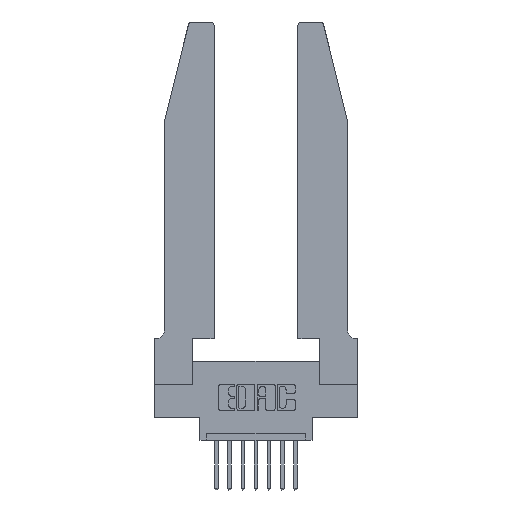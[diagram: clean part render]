
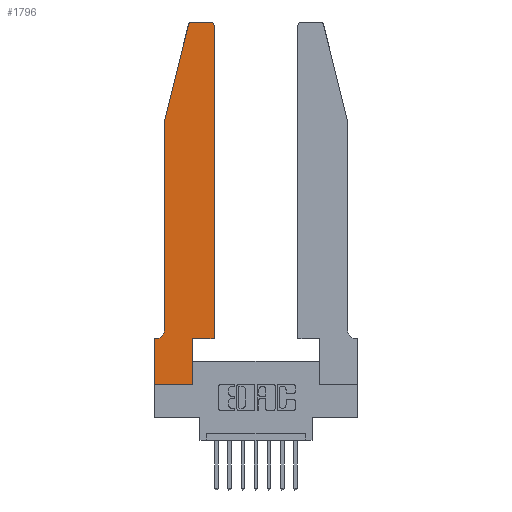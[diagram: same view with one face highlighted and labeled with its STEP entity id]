
A CAD part, top view. The second image highlights one B-rep face of the part: STEP entity #1796.
In plain terms, the highlighted planar face has unit normal (0, 0, 1).
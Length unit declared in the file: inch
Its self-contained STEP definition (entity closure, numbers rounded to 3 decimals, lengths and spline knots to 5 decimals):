
#229 = ORIENTED_EDGE ( 'NONE', *, *, #1550, .T. ) ;
#230 = DIRECTION ( 'NONE',  ( 1., 0., 0. ) ) ;
#375 = EDGE_CURVE ( 'NONE', #14135, #950, #12281, .T. ) ;
#395 = DIRECTION ( 'NONE',  ( 0., 1., 0. ) ) ;
#457 = AXIS2_PLACEMENT_3D ( 'NONE', #3667, #13935, #230 ) ;
#546 = CARTESIAN_POINT ( 'NONE',  ( 0.4505, 0.35, 0.37 ) ) ;
#648 = EDGE_CURVE ( 'NONE', #1232, #12059, #10456, .T. ) ;
#710 = ORIENTED_EDGE ( 'NONE', *, *, #1595, .T. ) ;
#726 = DIRECTION ( 'NONE',  ( 1., 0., 0. ) ) ;
#830 = CARTESIAN_POINT ( 'NONE',  ( 0.4505, 2.72, 0.37 ) ) ;
#925 = DIRECTION ( 'NONE',  ( 0., 0., -1. ) ) ;
#950 = VERTEX_POINT ( 'NONE', #11310 ) ;
#986 = DIRECTION ( 'NONE',  ( 1., 0., 0. ) ) ;
#1047 = DIRECTION ( 'NONE',  ( -1., 0., 0. ) ) ;
#1192 = DIRECTION ( 'NONE',  ( 0., -1., 0. ) ) ;
#1232 = VERTEX_POINT ( 'NONE', #3815 ) ;
#1277 = ORIENTED_EDGE ( 'NONE', *, *, #648, .T. ) ;
#1492 = PLANE ( 'NONE',  #457 ) ;
#1550 = EDGE_CURVE ( 'NONE', #12592, #5306, #10961, .T. ) ;
#1595 = EDGE_CURVE ( 'NONE', #950, #5706, #12934, .T. ) ;
#1796 = ADVANCED_FACE ( 'NONE', ( #2168 ), #1492, .T. ) ;
#1823 = DIRECTION ( 'NONE',  ( -1., 0., 0. ) ) ;
#1862 = EDGE_CURVE ( 'NONE', #3837, #14767, #1971, .T. ) ;
#1971 = CIRCLE ( 'NONE', #5374, 0.03 ) ;
#2168 = FACE_OUTER_BOUND ( 'NONE', #11415, .T. ) ;
#2303 = CARTESIAN_POINT ( 'NONE',  ( 0.284, 2.75, 0.37 ) ) ;
#2706 = DIRECTION ( 'NONE',  ( 0., 0., 1. ) ) ;
#2870 = ORIENTED_EDGE ( 'NONE', *, *, #4803, .T. ) ;
#2921 = LINE ( 'NONE', #11728, #12466 ) ;
#3088 = CIRCLE ( 'NONE', #8132, 0.07 ) ;
#3297 = VECTOR ( 'NONE', #1823, 39.37008 ) ;
#3367 = VECTOR ( 'NONE', #726, 39.37008 ) ;
#3453 = EDGE_CURVE ( 'NONE', #5306, #11946, #10013, .T. ) ;
#3667 = CARTESIAN_POINT ( 'NONE',  ( 0., 0.35, 0.37 ) ) ;
#3739 = DIRECTION ( 'NONE',  ( -0.239, -0.971, 0. ) ) ;
#3809 = VECTOR ( 'NONE', #3739, 39.37008 ) ;
#3815 = CARTESIAN_POINT ( 'NONE',  ( 0.25487, 2.72718, 0.37 ) ) ;
#3837 = VERTEX_POINT ( 'NONE', #830 ) ;
#3891 = ORIENTED_EDGE ( 'NONE', *, *, #8938, .T. ) ;
#4136 = VECTOR ( 'NONE', #8651, 39.37008 ) ;
#4215 = CIRCLE ( 'NONE', #12086, 0.03 ) ;
#4458 = DIRECTION ( 'NONE',  ( 1., 0., 0. ) ) ;
#4609 = ORIENTED_EDGE ( 'NONE', *, *, #3453, .T. ) ;
#4619 = VECTOR ( 'NONE', #395, 39.37008 ) ;
#4803 = EDGE_CURVE ( 'NONE', #11946, #3837, #7689, .T. ) ;
#4971 = LINE ( 'NONE', #10014, #3367 ) ;
#5232 = ORIENTED_EDGE ( 'NONE', *, *, #13812, .T. ) ;
#5306 = VERTEX_POINT ( 'NONE', #6312 ) ;
#5374 = AXIS2_PLACEMENT_3D ( 'NONE', #14140, #2706, #6211 ) ;
#5556 = CARTESIAN_POINT ( 'NONE',  ( 0.4505, 0.35, 0.37 ) ) ;
#5706 = VERTEX_POINT ( 'NONE', #10268 ) ;
#5833 = VERTEX_POINT ( 'NONE', #10664 ) ;
#6033 = CARTESIAN_POINT ( 'NONE',  ( 0.0755, 2., 0.37 ) ) ;
#6211 = DIRECTION ( 'NONE',  ( 1., 0., 0. ) ) ;
#6312 = CARTESIAN_POINT ( 'NONE',  ( 0.2865, 0.35, 0.37 ) ) ;
#6602 = VECTOR ( 'NONE', #986, 39.37008 ) ;
#6753 = VERTEX_POINT ( 'NONE', #2303 ) ;
#6774 = ORIENTED_EDGE ( 'NONE', *, *, #1862, .T. ) ;
#6819 = CARTESIAN_POINT ( 'NONE',  ( 0., 0., 0.37 ) ) ;
#7458 = CARTESIAN_POINT ( 'NONE',  ( 0.2865, 0., 0.37 ) ) ;
#7612 = EDGE_CURVE ( 'NONE', #14767, #6753, #10496, .T. ) ;
#7613 = EDGE_CURVE ( 'NONE', #6753, #1232, #4215, .T. ) ;
#7689 = LINE ( 'NONE', #546, #4619 ) ;
#8132 = AXIS2_PLACEMENT_3D ( 'NONE', #8798, #925, #14589 ) ;
#8651 = DIRECTION ( 'NONE',  ( 0., 1., 0. ) ) ;
#8798 = CARTESIAN_POINT ( 'NONE',  ( 0.0055, 0.42, 0.37 ) ) ;
#8938 = EDGE_CURVE ( 'NONE', #12059, #5833, #2921, .T. ) ;
#9040 = CARTESIAN_POINT ( 'NONE',  ( 0.2605, 2.75, 0.37 ) ) ;
#10013 = LINE ( 'NONE', #5556, #6602 ) ;
#10014 = CARTESIAN_POINT ( 'NONE',  ( 0., 0., 0.37 ) ) ;
#10268 = CARTESIAN_POINT ( 'NONE',  ( 0., 0., 0.37 ) ) ;
#10456 = LINE ( 'NONE', #10603, #3809 ) ;
#10496 = LINE ( 'NONE', #9040, #13537 ) ;
#10549 = DIRECTION ( 'NONE',  ( 0., -1., 0. ) ) ;
#10593 = CARTESIAN_POINT ( 'NONE',  ( 0.4205, 2.75, 0.37 ) ) ;
#10603 = CARTESIAN_POINT ( 'NONE',  ( 0.0755, 2., 0.37 ) ) ;
#10664 = CARTESIAN_POINT ( 'NONE',  ( 0.0755, 0.42, 0.37 ) ) ;
#10961 = LINE ( 'NONE', #11122, #4136 ) ;
#11122 = CARTESIAN_POINT ( 'NONE',  ( 0.2865, 0.35, 0.37 ) ) ;
#11310 = CARTESIAN_POINT ( 'NONE',  ( 0., 0.35, 0.37 ) ) ;
#11415 = EDGE_LOOP ( 'NONE', ( #13917, #12649, #1277, #3891, #12641, #14638, #710, #5232, #229, #4609, #2870, #6774 ) ) ;
#11583 = CARTESIAN_POINT ( 'NONE',  ( 0.0055, 0.35, 0.37 ) ) ;
#11728 = CARTESIAN_POINT ( 'NONE',  ( 0.0755, 2., 0.37 ) ) ;
#11755 = EDGE_CURVE ( 'NONE', #5833, #14135, #3088, .T. ) ;
#11946 = VERTEX_POINT ( 'NONE', #14866 ) ;
#12059 = VERTEX_POINT ( 'NONE', #6033 ) ;
#12086 = AXIS2_PLACEMENT_3D ( 'NONE', #14621, #13588, #4458 ) ;
#12281 = LINE ( 'NONE', #14443, #3297 ) ;
#12466 = VECTOR ( 'NONE', #10549, 39.37008 ) ;
#12592 = VERTEX_POINT ( 'NONE', #7458 ) ;
#12641 = ORIENTED_EDGE ( 'NONE', *, *, #11755, .T. ) ;
#12649 = ORIENTED_EDGE ( 'NONE', *, *, #7613, .T. ) ;
#12934 = LINE ( 'NONE', #6819, #14191 ) ;
#13537 = VECTOR ( 'NONE', #1047, 39.37008 ) ;
#13588 = DIRECTION ( 'NONE',  ( 0., 0., 1. ) ) ;
#13812 = EDGE_CURVE ( 'NONE', #5706, #12592, #4971, .T. ) ;
#13917 = ORIENTED_EDGE ( 'NONE', *, *, #7612, .T. ) ;
#13935 = DIRECTION ( 'NONE',  ( 0., 0., 1. ) ) ;
#14135 = VERTEX_POINT ( 'NONE', #11583 ) ;
#14140 = CARTESIAN_POINT ( 'NONE',  ( 0.4205, 2.72, 0.37 ) ) ;
#14191 = VECTOR ( 'NONE', #1192, 39.37008 ) ;
#14443 = CARTESIAN_POINT ( 'NONE',  ( 0.0755, 0.35, 0.37 ) ) ;
#14589 = DIRECTION ( 'NONE',  ( -1., 0., 0. ) ) ;
#14621 = CARTESIAN_POINT ( 'NONE',  ( 0.284, 2.72, 0.37 ) ) ;
#14638 = ORIENTED_EDGE ( 'NONE', *, *, #375, .T. ) ;
#14767 = VERTEX_POINT ( 'NONE', #10593 ) ;
#14866 = CARTESIAN_POINT ( 'NONE',  ( 0.4505, 0.35, 0.37 ) ) ;
